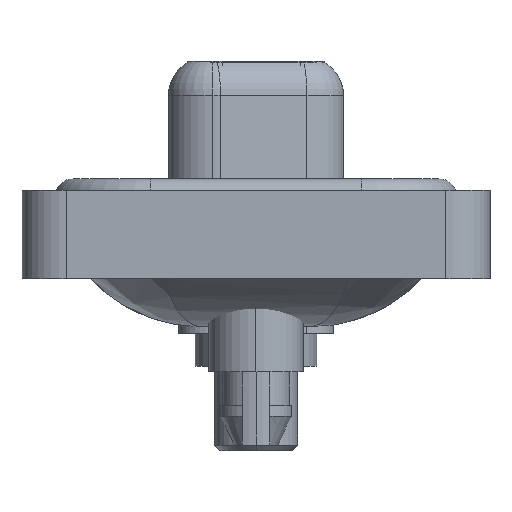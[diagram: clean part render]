
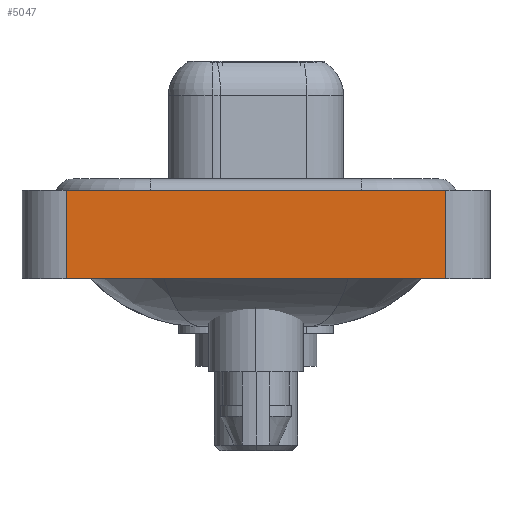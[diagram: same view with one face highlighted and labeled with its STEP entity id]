
A CAD part, left-side view. The second image highlights one B-rep face of the part: STEP entity #5047.
In plain terms, the highlighted planar face has unit normal (-1, 0, 0).
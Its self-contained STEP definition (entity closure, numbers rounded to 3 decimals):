
#65 = ORIENTED_EDGE ( 'NONE', *, *, #7936, .F. ) ;
#70 = ORIENTED_EDGE ( 'NONE', *, *, #11131, .T. ) ;
#99 = VERTEX_POINT ( 'NONE', #9193 ) ;
#416 = DIRECTION ( 'NONE',  ( 0., 0., 1. ) ) ;
#477 = DIRECTION ( 'NONE',  ( 0., 0., 1. ) ) ;
#929 = DIRECTION ( 'NONE',  ( 0., 0., 1. ) ) ;
#3405 = EDGE_LOOP ( 'NONE', ( #10081, #16977, #65, #70 ) ) ;
#3647 = CARTESIAN_POINT ( 'NONE',  ( -7.25, 8.55, 0.4 ) ) ;
#5047 = ADVANCED_FACE ( 'NONE', ( #10256 ), #7635, .T. ) ;
#5237 = VERTEX_POINT ( 'NONE', #3647 ) ;
#5394 = VECTOR ( 'NONE', #929, 1000. ) ;
#6120 = EDGE_CURVE ( 'NONE', #5237, #99, #17944, .T. ) ;
#7635 = PLANE ( 'NONE',  #12817 ) ;
#7812 = DIRECTION ( 'NONE',  ( 0., -1., 0. ) ) ;
#7936 = EDGE_CURVE ( 'NONE', #17890, #5237, #14571, .T. ) ;
#8005 = EDGE_CURVE ( 'NONE', #12121, #99, #9292, .T. ) ;
#9186 = LINE ( 'NONE', #13446, #10970 ) ;
#9193 = CARTESIAN_POINT ( 'NONE',  ( -7.25, -8.55, 0.4 ) ) ;
#9292 = LINE ( 'NONE', #13641, #5394 ) ;
#10081 = ORIENTED_EDGE ( 'NONE', *, *, #8005, .T. ) ;
#10256 = FACE_OUTER_BOUND ( 'NONE', #3405, .T. ) ;
#10871 = CARTESIAN_POINT ( 'NONE',  ( -7.25, -8.55, 0.4 ) ) ;
#10970 = VECTOR ( 'NONE', #11868, 1000. ) ;
#11020 = CARTESIAN_POINT ( 'NONE',  ( -7.25, 8.55, -3.6 ) ) ;
#11131 = EDGE_CURVE ( 'NONE', #17890, #12121, #9186, .T. ) ;
#11685 = CARTESIAN_POINT ( 'NONE',  ( -7.25, -8.55, -3.6 ) ) ;
#11868 = DIRECTION ( 'NONE',  ( 0., -1., 0. ) ) ;
#12121 = VERTEX_POINT ( 'NONE', #11685 ) ;
#12817 = AXIS2_PLACEMENT_3D ( 'NONE', #17498, #15902, #416 ) ;
#13188 = CARTESIAN_POINT ( 'NONE',  ( -7.25, 8.55, -3.6 ) ) ;
#13446 = CARTESIAN_POINT ( 'NONE',  ( -7.25, -8.55, -3.6 ) ) ;
#13641 = CARTESIAN_POINT ( 'NONE',  ( -7.25, -8.55, -3.6 ) ) ;
#14571 = LINE ( 'NONE', #13188, #15465 ) ;
#15465 = VECTOR ( 'NONE', #477, 1000. ) ;
#15902 = DIRECTION ( 'NONE',  ( -1., 0., 0. ) ) ;
#16389 = VECTOR ( 'NONE', #7812, 1000. ) ;
#16977 = ORIENTED_EDGE ( 'NONE', *, *, #6120, .F. ) ;
#17498 = CARTESIAN_POINT ( 'NONE',  ( -7.25, -8.55, -3.6 ) ) ;
#17890 = VERTEX_POINT ( 'NONE', #11020 ) ;
#17944 = LINE ( 'NONE', #10871, #16389 ) ;
